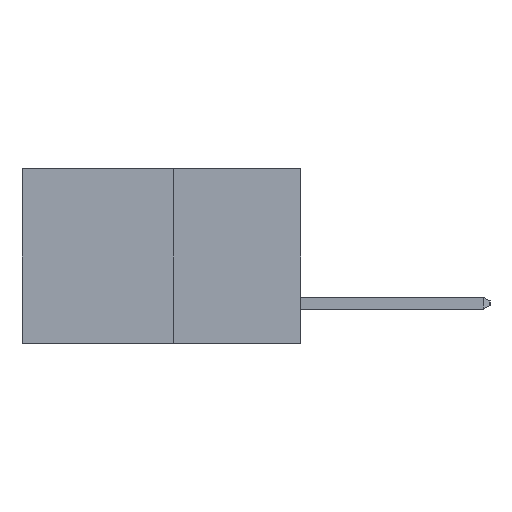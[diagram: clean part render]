
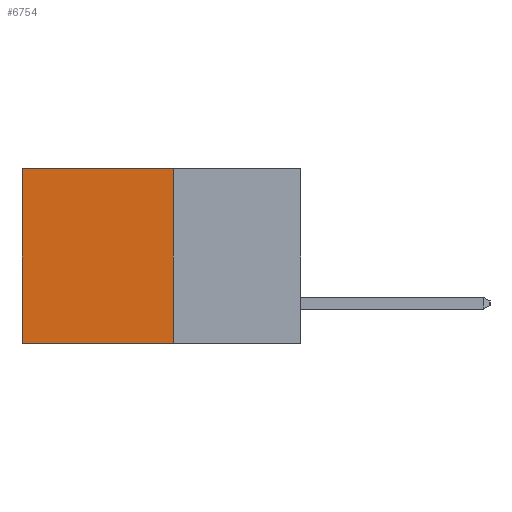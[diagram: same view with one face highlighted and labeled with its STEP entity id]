
A CAD part, left-side view. The second image highlights one B-rep face of the part: STEP entity #6754.
In plain terms, the highlighted planar face has unit normal (-1, 0, 0).
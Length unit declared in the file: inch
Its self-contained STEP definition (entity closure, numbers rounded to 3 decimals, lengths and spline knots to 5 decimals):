
#60 = CARTESIAN_POINT ( 'NONE',  ( 0.277, 0.27, -0.37 ) ) ;
#163 = LINE ( 'NONE', #403, #8977 ) ;
#363 = VERTEX_POINT ( 'NONE', #9477 ) ;
#403 = CARTESIAN_POINT ( 'NONE',  ( 0.277, 0.27, -0.37 ) ) ;
#549 = EDGE_LOOP ( 'NONE', ( #6199, #1217, #4885, #5132 ) ) ;
#808 = EDGE_CURVE ( 'NONE', #6615, #363, #10242, .T. ) ;
#1013 = DIRECTION ( 'NONE',  ( 1., 0., 0. ) ) ;
#1217 = ORIENTED_EDGE ( 'NONE', *, *, #6356, .F. ) ;
#2631 = FACE_OUTER_BOUND ( 'NONE', #549, .T. ) ;
#2950 = VERTEX_POINT ( 'NONE', #6891 ) ;
#3421 = DIRECTION ( 'NONE',  ( 0., 0., -1. ) ) ;
#3482 = VERTEX_POINT ( 'NONE', #8396 ) ;
#3985 = VECTOR ( 'NONE', #7817, 39.37008 ) ;
#4885 = ORIENTED_EDGE ( 'NONE', *, *, #7447, .F. ) ;
#5132 = ORIENTED_EDGE ( 'NONE', *, *, #5234, .T. ) ;
#5234 = EDGE_CURVE ( 'NONE', #3482, #6615, #8880, .T. ) ;
#6199 = ORIENTED_EDGE ( 'NONE', *, *, #808, .T. ) ;
#6356 = EDGE_CURVE ( 'NONE', #2950, #363, #163, .T. ) ;
#6615 = VERTEX_POINT ( 'NONE', #8477 ) ;
#6728 = VECTOR ( 'NONE', #7584, 39.37008 ) ;
#6754 = ADVANCED_FACE ( 'NONE', ( #2631 ), #6976, .F. ) ;
#6784 = CARTESIAN_POINT ( 'NONE',  ( 0.277, 0.27, 0. ) ) ;
#6891 = CARTESIAN_POINT ( 'NONE',  ( 0.277, 0.27, -0.37 ) ) ;
#6976 = PLANE ( 'NONE',  #10724 ) ;
#7004 = DIRECTION ( 'NONE',  ( 0., 0., -1. ) ) ;
#7447 = EDGE_CURVE ( 'NONE', #3482, #2950, #10393, .T. ) ;
#7584 = DIRECTION ( 'NONE',  ( 0., 1., 0. ) ) ;
#7817 = DIRECTION ( 'NONE',  ( 0., 0., -1. ) ) ;
#8103 = DIRECTION ( 'NONE',  ( 0., 1., 0. ) ) ;
#8155 = VECTOR ( 'NONE', #3421, 39.37008 ) ;
#8396 = CARTESIAN_POINT ( 'NONE',  ( 0.277, 0.27, 0. ) ) ;
#8477 = CARTESIAN_POINT ( 'NONE',  ( 0.277, 0.59, 0. ) ) ;
#8880 = LINE ( 'NONE', #6784, #6728 ) ;
#8977 = VECTOR ( 'NONE', #8103, 39.37008 ) ;
#9404 = CARTESIAN_POINT ( 'NONE',  ( 0.277, 0.27, -0.37 ) ) ;
#9477 = CARTESIAN_POINT ( 'NONE',  ( 0.277, 0.59, -0.37 ) ) ;
#9931 = CARTESIAN_POINT ( 'NONE',  ( 0.277, 0.59, -0.37 ) ) ;
#10242 = LINE ( 'NONE', #9931, #8155 ) ;
#10393 = LINE ( 'NONE', #9404, #3985 ) ;
#10724 = AXIS2_PLACEMENT_3D ( 'NONE', #60, #1013, #7004 ) ;
